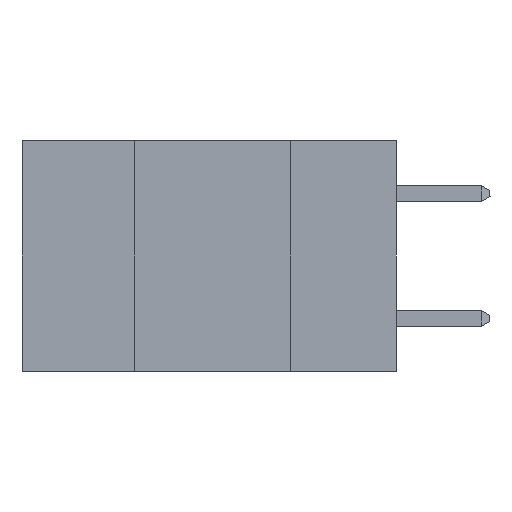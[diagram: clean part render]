
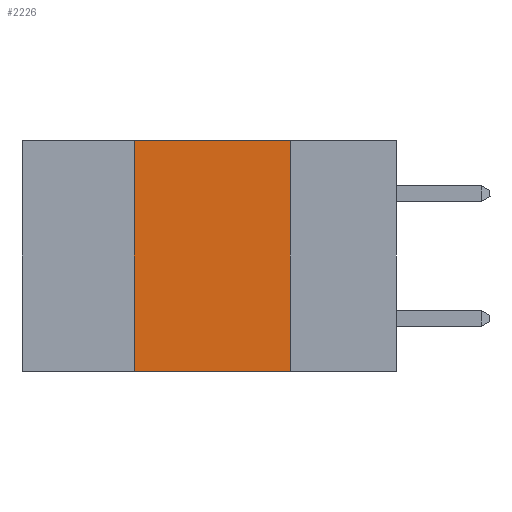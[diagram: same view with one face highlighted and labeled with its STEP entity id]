
A CAD part, left-side view. The second image highlights one B-rep face of the part: STEP entity #2226.
In plain terms, the highlighted planar face has unit normal (-1, 0, 0).
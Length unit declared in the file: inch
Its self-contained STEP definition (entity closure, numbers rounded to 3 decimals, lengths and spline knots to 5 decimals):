
#398 = VERTEX_POINT ( 'NONE', #23289 ) ;
#969 = EDGE_CURVE ( 'NONE', #15750, #21949, #11306, .T. ) ;
#2226 = ADVANCED_FACE ( 'NONE', ( #4697 ), #18589, .F. ) ;
#3224 = CARTESIAN_POINT ( 'NONE',  ( 0., 0.6, 0. ) ) ;
#3461 = ORIENTED_EDGE ( 'NONE', *, *, #969, .T. ) ;
#4697 = FACE_OUTER_BOUND ( 'NONE', #11484, .T. ) ;
#5004 = ORIENTED_EDGE ( 'NONE', *, *, #16529, .F. ) ;
#5395 = VECTOR ( 'NONE', #14832, 39.37008 ) ;
#5435 = CARTESIAN_POINT ( 'NONE',  ( 0., 0.42, -0.37 ) ) ;
#5829 = DIRECTION ( 'NONE',  ( 0., 0., -1. ) ) ;
#6744 = VECTOR ( 'NONE', #7238, 39.37008 ) ;
#7238 = DIRECTION ( 'NONE',  ( 0., -1., 0. ) ) ;
#7339 = EDGE_CURVE ( 'NONE', #398, #24333, #22487, .T. ) ;
#7779 = CARTESIAN_POINT ( 'NONE',  ( 0., 0.42, 0. ) ) ;
#9766 = CARTESIAN_POINT ( 'NONE',  ( 0., 0.17, 0. ) ) ;
#11306 = LINE ( 'NONE', #23834, #5395 ) ;
#11484 = EDGE_LOOP ( 'NONE', ( #18436, #24111, #5004, #3461 ) ) ;
#12060 = AXIS2_PLACEMENT_3D ( 'NONE', #12917, #13097, #17260 ) ;
#12917 = CARTESIAN_POINT ( 'NONE',  ( 0., 0.6, 0. ) ) ;
#13097 = DIRECTION ( 'NONE',  ( 1., 0., 0. ) ) ;
#13778 = DIRECTION ( 'NONE',  ( 0., 0., 1. ) ) ;
#14832 = DIRECTION ( 'NONE',  ( 0., -1., 0. ) ) ;
#15183 = EDGE_CURVE ( 'NONE', #24333, #21949, #25055, .T. ) ;
#15750 = VERTEX_POINT ( 'NONE', #5435 ) ;
#16208 = CARTESIAN_POINT ( 'NONE',  ( 0., 0.17, 0. ) ) ;
#16529 = EDGE_CURVE ( 'NONE', #15750, #398, #23769, .T. ) ;
#17260 = DIRECTION ( 'NONE',  ( 0., 0., -1. ) ) ;
#18071 = VECTOR ( 'NONE', #13778, 39.37008 ) ;
#18436 = ORIENTED_EDGE ( 'NONE', *, *, #15183, .F. ) ;
#18589 = PLANE ( 'NONE',  #12060 ) ;
#19988 = VECTOR ( 'NONE', #5829, 39.37008 ) ;
#20969 = CARTESIAN_POINT ( 'NONE',  ( 0., 0.17, -0.37 ) ) ;
#21949 = VERTEX_POINT ( 'NONE', #20969 ) ;
#22487 = LINE ( 'NONE', #3224, #6744 ) ;
#23289 = CARTESIAN_POINT ( 'NONE',  ( 0., 0.42, 0. ) ) ;
#23769 = LINE ( 'NONE', #7779, #18071 ) ;
#23834 = CARTESIAN_POINT ( 'NONE',  ( 0., 0.6, -0.37 ) ) ;
#24111 = ORIENTED_EDGE ( 'NONE', *, *, #7339, .F. ) ;
#24333 = VERTEX_POINT ( 'NONE', #16208 ) ;
#25055 = LINE ( 'NONE', #9766, #19988 ) ;
